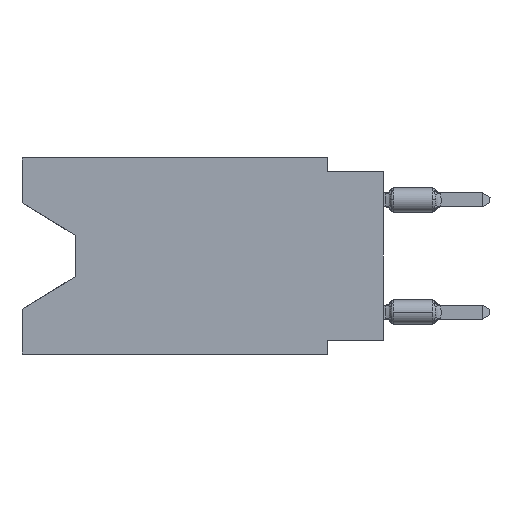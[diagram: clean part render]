
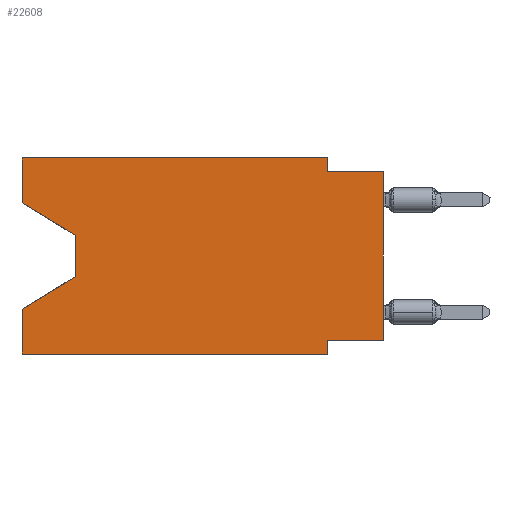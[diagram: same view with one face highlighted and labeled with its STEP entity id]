
A CAD part, left-side view. The second image highlights one B-rep face of the part: STEP entity #22608.
In plain terms, the highlighted planar face has unit normal (-1, 0, 0).
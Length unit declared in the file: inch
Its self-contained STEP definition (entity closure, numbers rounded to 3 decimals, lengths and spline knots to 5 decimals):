
#73 = CARTESIAN_POINT ( 'NONE',  ( 0., 0.645, -0.08025 ) ) ;
#85 = VECTOR ( 'NONE', #19561, 39.37008 ) ;
#175 = EDGE_CURVE ( 'NONE', #16123, #23058, #8280, .T. ) ;
#398 = CARTESIAN_POINT ( 'NONE',  ( 0., 0.55, -0.212 ) ) ;
#699 = EDGE_CURVE ( 'NONE', #10448, #3045, #4498, .T. ) ;
#786 = PLANE ( 'NONE',  #3412 ) ;
#1446 = ORIENTED_EDGE ( 'NONE', *, *, #14505, .F. ) ;
#2143 = VECTOR ( 'NONE', #21976, 39.37008 ) ;
#2455 = CARTESIAN_POINT ( 'NONE',  ( 0., 0.1, 0. ) ) ;
#3015 = EDGE_CURVE ( 'NONE', #23058, #23905, #26764, .T. ) ;
#3045 = VERTEX_POINT ( 'NONE', #26627 ) ;
#3288 = LINE ( 'NONE', #11993, #19356 ) ;
#3412 = AXIS2_PLACEMENT_3D ( 'NONE', #24582, #13755, #26598 ) ;
#4356 = VECTOR ( 'NONE', #7253, 39.37008 ) ;
#4498 = LINE ( 'NONE', #21873, #13856 ) ;
#5468 = VERTEX_POINT ( 'NONE', #23046 ) ;
#6021 = LINE ( 'NONE', #27975, #10401 ) ;
#6642 = LINE ( 'NONE', #73, #10253 ) ;
#6715 = DIRECTION ( 'NONE',  ( 0., 0., -1. ) ) ;
#6747 = LINE ( 'NONE', #2455, #2143 ) ;
#7253 = DIRECTION ( 'NONE',  ( 0., 0., 1. ) ) ;
#7541 = LINE ( 'NONE', #24918, #26454 ) ;
#7737 = ORIENTED_EDGE ( 'NONE', *, *, #23396, .F. ) ;
#8147 = EDGE_CURVE ( 'NONE', #24778, #16123, #6642, .T. ) ;
#8280 = LINE ( 'NONE', #14564, #12560 ) ;
#8684 = CARTESIAN_POINT ( 'NONE',  ( 0., 0., -0.325 ) ) ;
#8787 = EDGE_CURVE ( 'NONE', #10448, #23905, #3288, .T. ) ;
#8919 = ORIENTED_EDGE ( 'NONE', *, *, #8147, .T. ) ;
#9455 = CARTESIAN_POINT ( 'NONE',  ( 0., 0.55, -0.212 ) ) ;
#10253 = VECTOR ( 'NONE', #15468, 39.37008 ) ;
#10260 = VECTOR ( 'NONE', #15212, 39.37008 ) ;
#10401 = VECTOR ( 'NONE', #25689, 39.37008 ) ;
#10448 = VERTEX_POINT ( 'NONE', #14006 ) ;
#10786 = VERTEX_POINT ( 'NONE', #15018 ) ;
#10882 = EDGE_CURVE ( 'NONE', #13155, #26891, #6747, .T. ) ;
#11064 = DIRECTION ( 'NONE',  ( 0., -1., 0. ) ) ;
#11993 = CARTESIAN_POINT ( 'NONE',  ( 0., 0.645, 0. ) ) ;
#12453 = CARTESIAN_POINT ( 'NONE',  ( 0., 0.1, 0. ) ) ;
#12560 = VECTOR ( 'NONE', #27380, 39.37008 ) ;
#12913 = ORIENTED_EDGE ( 'NONE', *, *, #13713, .F. ) ;
#12954 = CARTESIAN_POINT ( 'NONE',  ( 0., 0.55, -0.138 ) ) ;
#13155 = VERTEX_POINT ( 'NONE', #12453 ) ;
#13623 = FACE_OUTER_BOUND ( 'NONE', #18830, .T. ) ;
#13676 = CARTESIAN_POINT ( 'NONE',  ( 0., 0.1, -0.35 ) ) ;
#13713 = EDGE_CURVE ( 'NONE', #26891, #5468, #7541, .T. ) ;
#13755 = DIRECTION ( 'NONE',  ( 1., 0., 0. ) ) ;
#13856 = VECTOR ( 'NONE', #11064, 39.37008 ) ;
#13990 = DIRECTION ( 'NONE',  ( 0., 0., 1. ) ) ;
#14006 = CARTESIAN_POINT ( 'NONE',  ( 0., 0.645, -0.35 ) ) ;
#14092 = DIRECTION ( 'NONE',  ( 0., -1., 0. ) ) ;
#14256 = VECTOR ( 'NONE', #6715, 39.37008 ) ;
#14505 = EDGE_CURVE ( 'NONE', #17449, #25486, #22387, .T. ) ;
#14564 = CARTESIAN_POINT ( 'NONE',  ( 0., 0.55, -0.138 ) ) ;
#14867 = CARTESIAN_POINT ( 'NONE',  ( 0., 0.1, -0.025 ) ) ;
#14921 = ORIENTED_EDGE ( 'NONE', *, *, #17814, .F. ) ;
#15018 = CARTESIAN_POINT ( 'NONE',  ( 0., 0.645, 0. ) ) ;
#15208 = ORIENTED_EDGE ( 'NONE', *, *, #699, .T. ) ;
#15212 = DIRECTION ( 'NONE',  ( 0., -1., 0. ) ) ;
#15401 = LINE ( 'NONE', #13676, #14256 ) ;
#15468 = DIRECTION ( 'NONE',  ( 0., -0.855, -0.519 ) ) ;
#15761 = EDGE_CURVE ( 'NONE', #25486, #3045, #15401, .T. ) ;
#16063 = DIRECTION ( 'NONE',  ( 0., 0.855, -0.519 ) ) ;
#16123 = VERTEX_POINT ( 'NONE', #12954 ) ;
#16144 = CARTESIAN_POINT ( 'NONE',  ( 0., 0.645, -0.08025 ) ) ;
#16287 = ORIENTED_EDGE ( 'NONE', *, *, #15761, .F. ) ;
#16939 = ORIENTED_EDGE ( 'NONE', *, *, #26843, .T. ) ;
#17224 = CARTESIAN_POINT ( 'NONE',  ( 0., 0.645, 0. ) ) ;
#17251 = ORIENTED_EDGE ( 'NONE', *, *, #3015, .T. ) ;
#17449 = VERTEX_POINT ( 'NONE', #8684 ) ;
#17814 = EDGE_CURVE ( 'NONE', #10786, #13155, #25901, .T. ) ;
#17901 = CARTESIAN_POINT ( 'NONE',  ( 0., 0.1, -0.325 ) ) ;
#18639 = CARTESIAN_POINT ( 'NONE',  ( 0., 0.645, 0. ) ) ;
#18830 = EDGE_LOOP ( 'NONE', ( #8919, #27830, #17251, #24907, #15208, #16287, #1446, #16939, #12913, #19435, #14921, #7737 ) ) ;
#19356 = VECTOR ( 'NONE', #13990, 39.37008 ) ;
#19435 = ORIENTED_EDGE ( 'NONE', *, *, #10882, .F. ) ;
#19561 = DIRECTION ( 'NONE',  ( 0., 1., 0. ) ) ;
#20739 = CARTESIAN_POINT ( 'NONE',  ( 0., 0.645, -0.26975 ) ) ;
#21873 = CARTESIAN_POINT ( 'NONE',  ( 0., 0.645, -0.35 ) ) ;
#21976 = DIRECTION ( 'NONE',  ( 0., 0., -1. ) ) ;
#22387 = LINE ( 'NONE', #26264, #85 ) ;
#22608 = ADVANCED_FACE ( 'NONE', ( #13623 ), #786, .F. ) ;
#23046 = CARTESIAN_POINT ( 'NONE',  ( 0., 0., -0.025 ) ) ;
#23058 = VERTEX_POINT ( 'NONE', #9455 ) ;
#23396 = EDGE_CURVE ( 'NONE', #24778, #10786, #26779, .T. ) ;
#23905 = VERTEX_POINT ( 'NONE', #20739 ) ;
#24581 = VECTOR ( 'NONE', #16063, 39.37008 ) ;
#24582 = CARTESIAN_POINT ( 'NONE',  ( 0., 0.645, 0. ) ) ;
#24778 = VERTEX_POINT ( 'NONE', #16144 ) ;
#24907 = ORIENTED_EDGE ( 'NONE', *, *, #8787, .F. ) ;
#24918 = CARTESIAN_POINT ( 'NONE',  ( 0., 0., -0.025 ) ) ;
#25486 = VERTEX_POINT ( 'NONE', #17901 ) ;
#25689 = DIRECTION ( 'NONE',  ( 0., 0., 1. ) ) ;
#25901 = LINE ( 'NONE', #17224, #10260 ) ;
#26264 = CARTESIAN_POINT ( 'NONE',  ( 0., 0., -0.325 ) ) ;
#26454 = VECTOR ( 'NONE', #14092, 39.37008 ) ;
#26598 = DIRECTION ( 'NONE',  ( 0., 0., -1. ) ) ;
#26627 = CARTESIAN_POINT ( 'NONE',  ( 0., 0.1, -0.35 ) ) ;
#26764 = LINE ( 'NONE', #398, #24581 ) ;
#26779 = LINE ( 'NONE', #18639, #4356 ) ;
#26843 = EDGE_CURVE ( 'NONE', #17449, #5468, #6021, .T. ) ;
#26891 = VERTEX_POINT ( 'NONE', #14867 ) ;
#27380 = DIRECTION ( 'NONE',  ( 0., 0., -1. ) ) ;
#27830 = ORIENTED_EDGE ( 'NONE', *, *, #175, .T. ) ;
#27975 = CARTESIAN_POINT ( 'NONE',  ( 0., 0., 0. ) ) ;
